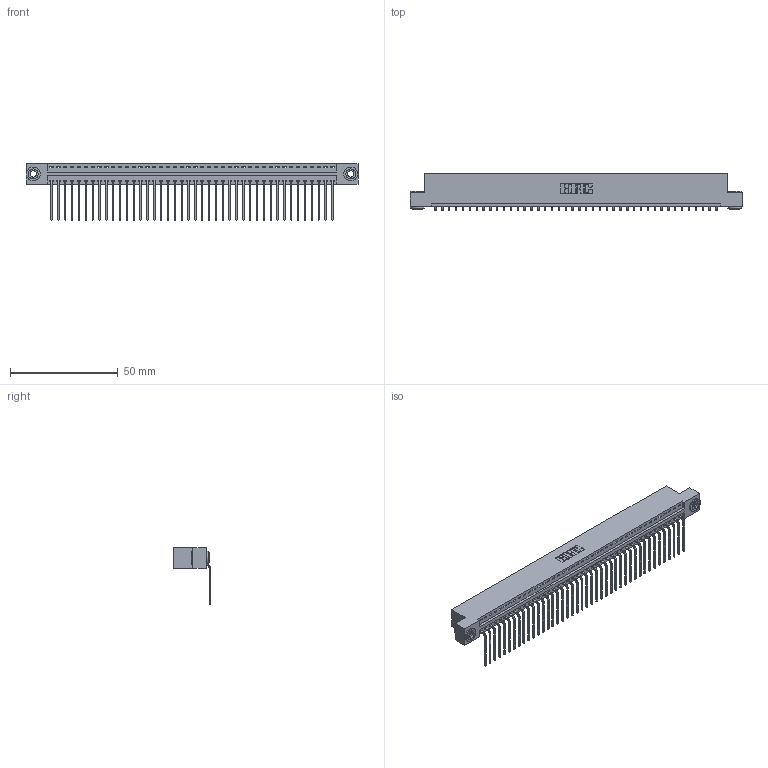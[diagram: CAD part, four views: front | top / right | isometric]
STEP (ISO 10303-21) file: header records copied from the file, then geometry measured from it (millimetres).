
FILE_DESCRIPTION (( 'STEP AP203' ), '1' );
FILE_NAME ('346-042-559-103.STEP', '2022-05-09T14:58:56', ( '' ), ( '' ), 'SwSTEP 2.0', 'SolidWorks 2020', '' );
FILE_SCHEMA (( 'CONFIG_CONTROL_DESIGN' ));
Length unit declared in the file: inch
Products named in the file (4): 346-042-559-103; 345-292-001_558 559 Tail - 1; 345-250-002_345-250-002-102; 346 Part_Flush Mounting Lugs - 0.156 Dia-TH
Assembly tree (45 placements, depth 2):
  346-042-559-103
    346 Part_Flush Mounting Lugs - 0.156 Dia-TH
    345-292-001_558 559 Tail - 1  x42
    345-250-002_345-250-002-102  x2
Bounding box: 153.92 x 17.08 x 26.16 mm (x, y, z)
Volume: 14875.2 mm3; surface area: 19678.3 mm2
Topology: 45 solids, 45 shells, 2694 faces, 8085 edges, 5330 vertices
Faces by surface type: plane 1864, cylinder 822, cone 8
Entity records: 27216 total; most frequent: CARTESIAN_POINT 4647, ORIENTED_EDGE 4614, DIRECTION 4129, EDGE_CURVE 2307, LINE 1983, VECTOR 1983, VERTEX_POINT 1534, AXIS2_PLACEMENT_3D 1073
